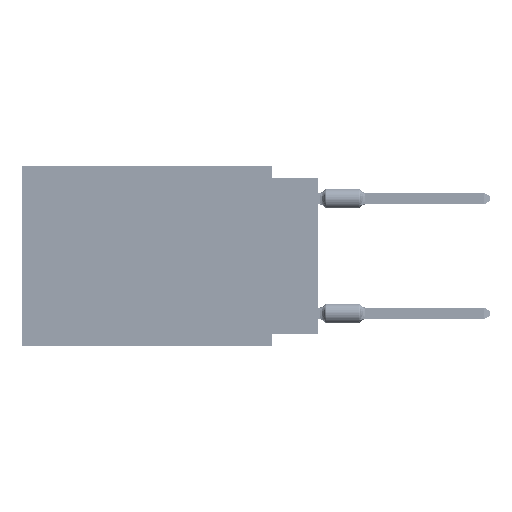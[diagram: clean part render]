
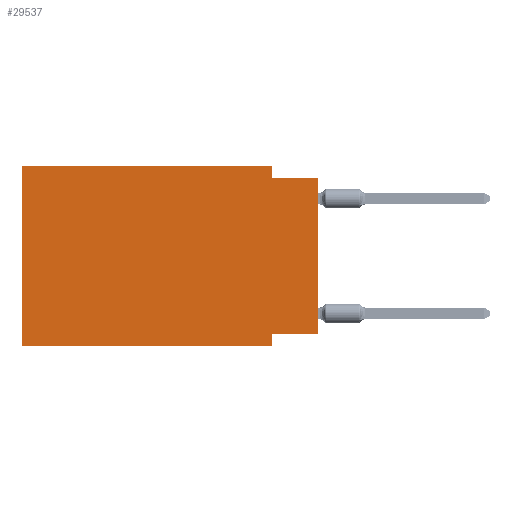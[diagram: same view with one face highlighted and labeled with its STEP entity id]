
A CAD part, left-side view. The second image highlights one B-rep face of the part: STEP entity #29537.
In plain terms, the highlighted planar face has unit normal (-1, 0, 0).
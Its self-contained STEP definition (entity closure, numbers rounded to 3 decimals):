
#235 = CARTESIAN_POINT ( 'NONE',  ( 0., 16.383, 0. ) ) ;
#328 = VERTEX_POINT ( 'NONE', #52803 ) ;
#674 = EDGE_LOOP ( 'NONE', ( #67054, #29279, #58620, #36492, #26187, #7640, #38543, #20943 ) ) ;
#1239 = CARTESIAN_POINT ( 'NONE',  ( 0., 2.54, 0. ) ) ;
#4012 = VERTEX_POINT ( 'NONE', #50047 ) ;
#4710 = DIRECTION ( 'NONE',  ( 0., -1., 0. ) ) ;
#4769 = VERTEX_POINT ( 'NONE', #7639 ) ;
#5253 = PLANE ( 'NONE',  #27600 ) ;
#7639 = CARTESIAN_POINT ( 'NONE',  ( 0., 16.383, -9.906 ) ) ;
#7640 = ORIENTED_EDGE ( 'NONE', *, *, #9580, .T. ) ;
#9580 = EDGE_CURVE ( 'NONE', #4769, #4012, #60051, .T. ) ;
#15481 = EDGE_CURVE ( 'NONE', #39221, #328, #21459, .T. ) ;
#15864 = CARTESIAN_POINT ( 'NONE',  ( 0., 0., -0.635 ) ) ;
#16395 = EDGE_CURVE ( 'NONE', #17211, #4012, #60375, .T. ) ;
#17088 = FACE_OUTER_BOUND ( 'NONE', #674, .T. ) ;
#17211 = VERTEX_POINT ( 'NONE', #60471 ) ;
#17764 = CARTESIAN_POINT ( 'NONE',  ( 0., 2.54, -9.906 ) ) ;
#20943 = ORIENTED_EDGE ( 'NONE', *, *, #41228, .F. ) ;
#21459 = LINE ( 'NONE', #15864, #55245 ) ;
#22006 = CARTESIAN_POINT ( 'NONE',  ( 0., 16.383, 0. ) ) ;
#22208 = LINE ( 'NONE', #1239, #66992 ) ;
#24887 = VERTEX_POINT ( 'NONE', #24928 ) ;
#24928 = CARTESIAN_POINT ( 'NONE',  ( 0., 0., -9.271 ) ) ;
#25434 = EDGE_CURVE ( 'NONE', #24887, #328, #47164, .T. ) ;
#25659 = CARTESIAN_POINT ( 'NONE',  ( 0., 0., -9.271 ) ) ;
#26187 = ORIENTED_EDGE ( 'NONE', *, *, #40558, .F. ) ;
#26283 = VECTOR ( 'NONE', #68477, 1000. ) ;
#27589 = CARTESIAN_POINT ( 'NONE',  ( 0., 16.383, -9.906 ) ) ;
#27600 = AXIS2_PLACEMENT_3D ( 'NONE', #22006, #43634, #59355 ) ;
#28705 = CARTESIAN_POINT ( 'NONE',  ( 0., 2.54, 0. ) ) ;
#29279 = ORIENTED_EDGE ( 'NONE', *, *, #15481, .F. ) ;
#29537 = ADVANCED_FACE ( 'NONE', ( #17088 ), #5253, .F. ) ;
#33830 = DIRECTION ( 'NONE',  ( 0., 0., -1. ) ) ;
#36211 = LINE ( 'NONE', #235, #59257 ) ;
#36492 = ORIENTED_EDGE ( 'NONE', *, *, #46246, .F. ) ;
#36811 = DIRECTION ( 'NONE',  ( 0., 1., 0. ) ) ;
#38317 = CARTESIAN_POINT ( 'NONE',  ( 0., 16.383, 0. ) ) ;
#38543 = ORIENTED_EDGE ( 'NONE', *, *, #16395, .F. ) ;
#39221 = VERTEX_POINT ( 'NONE', #46338 ) ;
#39333 = EDGE_CURVE ( 'NONE', #62076, #39221, #22208, .T. ) ;
#40558 = EDGE_CURVE ( 'NONE', #4769, #64042, #36211, .T. ) ;
#41228 = EDGE_CURVE ( 'NONE', #24887, #17211, #53569, .T. ) ;
#42586 = DIRECTION ( 'NONE',  ( 0., -1., 0. ) ) ;
#43634 = DIRECTION ( 'NONE',  ( 1., 0., 0. ) ) ;
#46246 = EDGE_CURVE ( 'NONE', #64042, #62076, #49191, .T. ) ;
#46338 = CARTESIAN_POINT ( 'NONE',  ( 0., 2.54, -0.635 ) ) ;
#47037 = DIRECTION ( 'NONE',  ( 0., 0., 1. ) ) ;
#47164 = LINE ( 'NONE', #67093, #26283 ) ;
#48853 = CARTESIAN_POINT ( 'NONE',  ( 0., 16.383, 0. ) ) ;
#49191 = LINE ( 'NONE', #48853, #67456 ) ;
#49906 = DIRECTION ( 'NONE',  ( 0., -1., 0. ) ) ;
#50047 = CARTESIAN_POINT ( 'NONE',  ( 0., 2.54, -9.906 ) ) ;
#52685 = VECTOR ( 'NONE', #36811, 1000. ) ;
#52803 = CARTESIAN_POINT ( 'NONE',  ( 0., 0., -0.635 ) ) ;
#53569 = LINE ( 'NONE', #25659, #52685 ) ;
#55245 = VECTOR ( 'NONE', #4710, 1000. ) ;
#58620 = ORIENTED_EDGE ( 'NONE', *, *, #39333, .F. ) ;
#59257 = VECTOR ( 'NONE', #47037, 1000. ) ;
#59355 = DIRECTION ( 'NONE',  ( 0., 0., -1. ) ) ;
#60051 = LINE ( 'NONE', #27589, #65911 ) ;
#60375 = LINE ( 'NONE', #17764, #64284 ) ;
#60471 = CARTESIAN_POINT ( 'NONE',  ( 0., 2.54, -9.271 ) ) ;
#62076 = VERTEX_POINT ( 'NONE', #28705 ) ;
#64042 = VERTEX_POINT ( 'NONE', #38317 ) ;
#64284 = VECTOR ( 'NONE', #33830, 1000. ) ;
#64474 = DIRECTION ( 'NONE',  ( 0., 0., -1. ) ) ;
#65911 = VECTOR ( 'NONE', #49906, 1000. ) ;
#66992 = VECTOR ( 'NONE', #64474, 1000. ) ;
#67054 = ORIENTED_EDGE ( 'NONE', *, *, #25434, .T. ) ;
#67093 = CARTESIAN_POINT ( 'NONE',  ( 0., 0., 0. ) ) ;
#67456 = VECTOR ( 'NONE', #42586, 1000. ) ;
#68477 = DIRECTION ( 'NONE',  ( 0., 0., 1. ) ) ;
